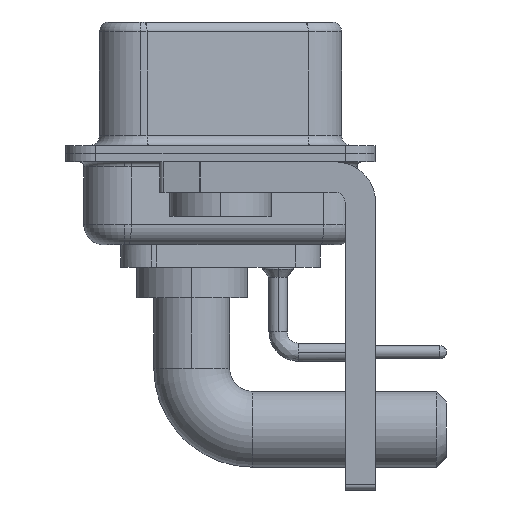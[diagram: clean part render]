
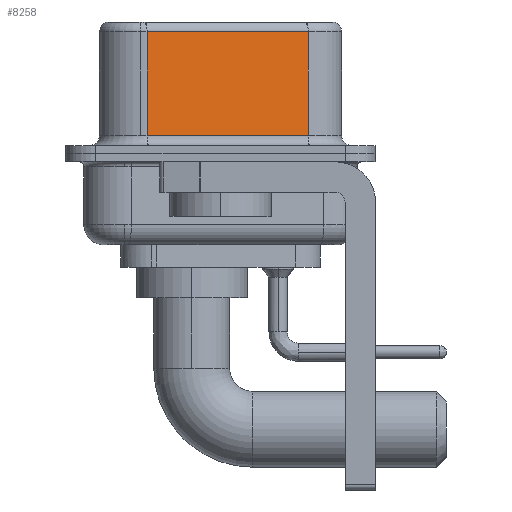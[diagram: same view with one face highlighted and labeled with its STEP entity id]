
A CAD part, left-side view. The second image highlights one B-rep face of the part: STEP entity #8258.
In plain terms, the highlighted planar face has unit normal (-0.985, -0.174, 0).
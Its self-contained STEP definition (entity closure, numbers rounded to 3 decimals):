
#1159 = DIRECTION ( 'NONE',  ( 0.174, -0.985, 0. ) ) ;
#1661 = FACE_OUTER_BOUND ( 'NONE', #12548, .T. ) ;
#1748 = DIRECTION ( 'NONE',  ( -0.174, 0.985, 0. ) ) ;
#1880 = CARTESIAN_POINT ( 'NONE',  ( 5.132, -4.322, 6.52 ) ) ;
#2026 = VECTOR ( 'NONE', #17205, 1000. ) ;
#2395 = CARTESIAN_POINT ( 'NONE',  ( 5.132, -4.322, 6.02 ) ) ;
#3325 = CARTESIAN_POINT ( 'NONE',  ( 5.132, -4.322, 0.9 ) ) ;
#3416 = VECTOR ( 'NONE', #13463, 1000. ) ;
#3442 = EDGE_CURVE ( 'NONE', #17375, #11517, #14947, .T. ) ;
#4444 = CARTESIAN_POINT ( 'NONE',  ( 3.73, 3.628, 0.9 ) ) ;
#4970 = ORIENTED_EDGE ( 'NONE', *, *, #12412, .T. ) ;
#7432 = CARTESIAN_POINT ( 'NONE',  ( 5.132, -4.322, 6.52 ) ) ;
#8258 = ADVANCED_FACE ( 'NONE', ( #1661 ), #16986, .F. ) ;
#9752 = LINE ( 'NONE', #15540, #18071 ) ;
#9780 = DIRECTION ( 'NONE',  ( -0.174, 0.985, 0. ) ) ;
#10190 = VERTEX_POINT ( 'NONE', #20350 ) ;
#11517 = VERTEX_POINT ( 'NONE', #13971 ) ;
#12107 = ORIENTED_EDGE ( 'NONE', *, *, #3442, .F. ) ;
#12313 = LINE ( 'NONE', #3325, #24108 ) ;
#12412 = EDGE_CURVE ( 'NONE', #17375, #10190, #9752, .T. ) ;
#12548 = EDGE_LOOP ( 'NONE', ( #12107, #4970, #21214, #19795 ) ) ;
#13463 = DIRECTION ( 'NONE',  ( 0., 0., -1. ) ) ;
#13971 = CARTESIAN_POINT ( 'NONE',  ( 5.132, -4.322, 0.9 ) ) ;
#14947 = LINE ( 'NONE', #1880, #2026 ) ;
#15013 = LINE ( 'NONE', #22681, #3416 ) ;
#15092 = DIRECTION ( 'NONE',  ( 0.985, 0.174, 0. ) ) ;
#15540 = CARTESIAN_POINT ( 'NONE',  ( 5.132, -4.322, 6.02 ) ) ;
#15565 = VERTEX_POINT ( 'NONE', #4444 ) ;
#16986 = PLANE ( 'NONE',  #23549 ) ;
#17162 = EDGE_CURVE ( 'NONE', #15565, #11517, #12313, .T. ) ;
#17205 = DIRECTION ( 'NONE',  ( 0., 0., -1. ) ) ;
#17375 = VERTEX_POINT ( 'NONE', #2395 ) ;
#18071 = VECTOR ( 'NONE', #1748, 1000. ) ;
#19795 = ORIENTED_EDGE ( 'NONE', *, *, #17162, .T. ) ;
#20350 = CARTESIAN_POINT ( 'NONE',  ( 3.73, 3.628, 6.02 ) ) ;
#21214 = ORIENTED_EDGE ( 'NONE', *, *, #21552, .T. ) ;
#21552 = EDGE_CURVE ( 'NONE', #10190, #15565, #15013, .T. ) ;
#22681 = CARTESIAN_POINT ( 'NONE',  ( 3.73, 3.628, 6.52 ) ) ;
#23549 = AXIS2_PLACEMENT_3D ( 'NONE', #7432, #15092, #9780 ) ;
#24108 = VECTOR ( 'NONE', #1159, 1000. ) ;
